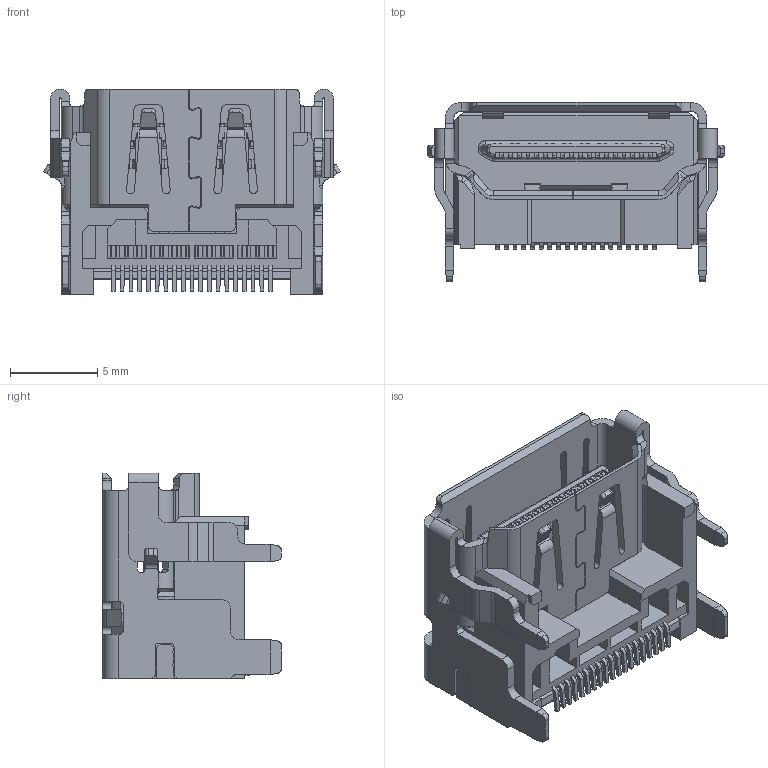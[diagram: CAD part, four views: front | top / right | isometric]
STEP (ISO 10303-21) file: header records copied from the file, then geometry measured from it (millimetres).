
FILE_DESCRIPTION (( 'STEP AP214' ), '1' );
FILE_NAME ('694D119-164-111.STEP', '2021-01-13T17:12:03', ( '' ), ( '' ), 'SwSTEP 2.0', 'SolidWorks 2020', '' );
FILE_SCHEMA (( 'AUTOMOTIVE_DESIGN' ));
Length unit declared in the file: millimetre
Products named in the file (5): 694D119-164-111; Insulator 694D119-X64-111; Contact Lower 694D119-X64-111; Shell 694D119-X64-111; Contact Upper 694D119-X64-111
Assembly tree (21 placements, depth 2):
  694D119-164-111
    Insulator 694D119-X64-111
    Contact Upper 694D119-X64-111  x10
    Contact Lower 694D119-X64-111  x9
    Shell 694D119-X64-111
Bounding box: 17.01 x 10.25 x 11.8 mm (x, y, z)
Volume: 550.3 mm3; surface area: 2217.9 mm2
Topology: 21 solids, 21 shells, 3276 faces, 9327 edges, 6055 vertices
Faces by surface type: plane 2261, cylinder 948, bspline 57, cone 10
Entity records: 71670 total; most frequent: CARTESIAN_POINT 15678, ORIENTED_EDGE 12212, DIRECTION 10783, EDGE_CURVE 6106, LINE 4739, VECTOR 4739, VERTEX_POINT 3913, AXIS2_PLACEMENT_3D 3022
